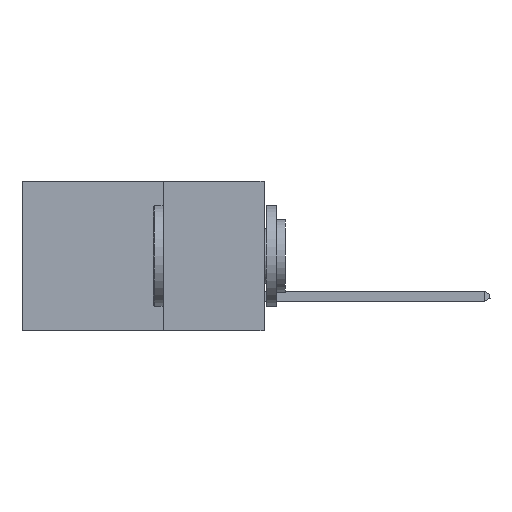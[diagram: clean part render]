
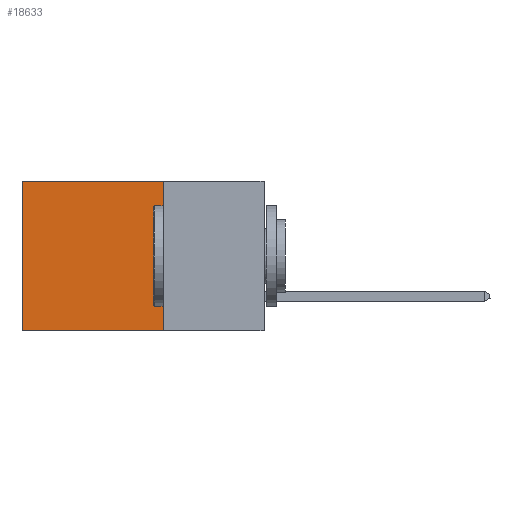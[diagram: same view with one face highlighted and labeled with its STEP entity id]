
A CAD part, left-side view. The second image highlights one B-rep face of the part: STEP entity #18633.
In plain terms, the highlighted planar face has unit normal (-1, 0, 0).
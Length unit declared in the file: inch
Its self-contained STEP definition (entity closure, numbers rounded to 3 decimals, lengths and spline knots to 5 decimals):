
#158 = DIRECTION ( 'NONE',  ( 0., 0., -1. ) ) ;
#482 = EDGE_LOOP ( 'NONE', ( #5326, #20534, #3021, #9013 ) ) ;
#1507 = DIRECTION ( 'NONE',  ( 0., 1., 0. ) ) ;
#1543 = LINE ( 'NONE', #6831, #2572 ) ;
#1926 = CARTESIAN_POINT ( 'NONE',  ( 0.298, 0.6, 0. ) ) ;
#1942 = DIRECTION ( 'NONE',  ( 0., 0., -1. ) ) ;
#2350 = VECTOR ( 'NONE', #11198, 39.37008 ) ;
#2572 = VECTOR ( 'NONE', #18340, 39.37008 ) ;
#2742 = LINE ( 'NONE', #16861, #15987 ) ;
#3021 = ORIENTED_EDGE ( 'NONE', *, *, #8981, .F. ) ;
#3138 = CARTESIAN_POINT ( 'NONE',  ( 0.298, 0.25, 0. ) ) ;
#3483 = VERTEX_POINT ( 'NONE', #15188 ) ;
#4245 = AXIS2_PLACEMENT_3D ( 'NONE', #18604, #13568, #158 ) ;
#4518 = CARTESIAN_POINT ( 'NONE',  ( 0.298, 0.25, 0. ) ) ;
#5326 = ORIENTED_EDGE ( 'NONE', *, *, #20608, .T. ) ;
#6227 = LINE ( 'NONE', #4518, #2350 ) ;
#6831 = CARTESIAN_POINT ( 'NONE',  ( 0.298, 0.25, 0. ) ) ;
#7029 = PLANE ( 'NONE',  #4245 ) ;
#7051 = VECTOR ( 'NONE', #1507, 39.37008 ) ;
#7718 = VERTEX_POINT ( 'NONE', #1926 ) ;
#8981 = EDGE_CURVE ( 'NONE', #12199, #13472, #1543, .T. ) ;
#9013 = ORIENTED_EDGE ( 'NONE', *, *, #14182, .T. ) ;
#11198 = DIRECTION ( 'NONE',  ( 0., 1., 0. ) ) ;
#11430 = CARTESIAN_POINT ( 'NONE',  ( 0.298, 0.25, -0.37 ) ) ;
#11474 = LINE ( 'NONE', #11430, #7051 ) ;
#12199 = VERTEX_POINT ( 'NONE', #3138 ) ;
#13472 = VERTEX_POINT ( 'NONE', #16104 ) ;
#13568 = DIRECTION ( 'NONE',  ( 1., 0., 0. ) ) ;
#13590 = EDGE_CURVE ( 'NONE', #13472, #3483, #11474, .T. ) ;
#14182 = EDGE_CURVE ( 'NONE', #12199, #7718, #6227, .T. ) ;
#15188 = CARTESIAN_POINT ( 'NONE',  ( 0.298, 0.6, -0.37 ) ) ;
#15987 = VECTOR ( 'NONE', #1942, 39.37008 ) ;
#16104 = CARTESIAN_POINT ( 'NONE',  ( 0.298, 0.25, -0.37 ) ) ;
#16367 = FACE_OUTER_BOUND ( 'NONE', #482, .T. ) ;
#16861 = CARTESIAN_POINT ( 'NONE',  ( 0.298, 0.6, 0. ) ) ;
#18340 = DIRECTION ( 'NONE',  ( 0., 0., -1. ) ) ;
#18604 = CARTESIAN_POINT ( 'NONE',  ( 0.298, 0.25, 0. ) ) ;
#18633 = ADVANCED_FACE ( 'NONE', ( #16367 ), #7029, .F. ) ;
#20534 = ORIENTED_EDGE ( 'NONE', *, *, #13590, .F. ) ;
#20608 = EDGE_CURVE ( 'NONE', #7718, #3483, #2742, .T. ) ;
